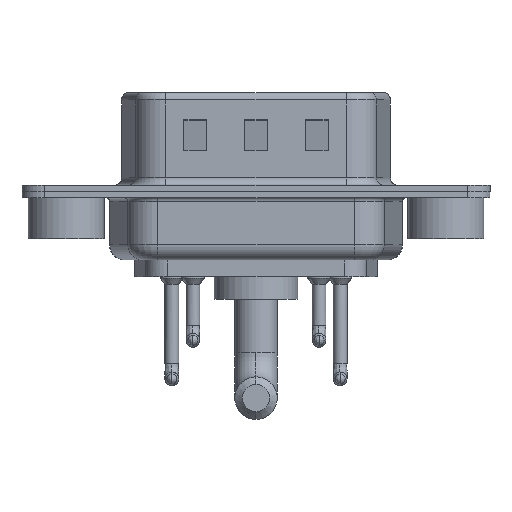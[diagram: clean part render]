
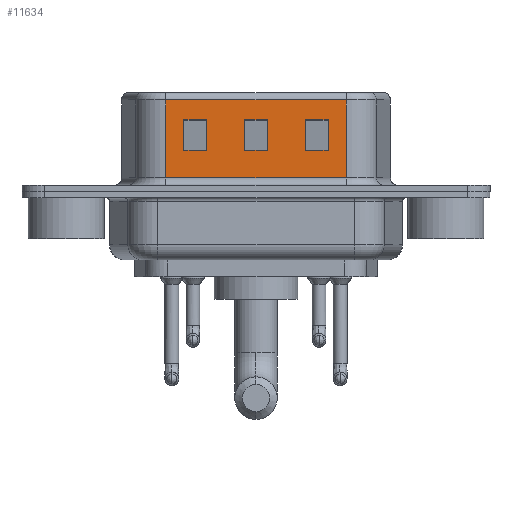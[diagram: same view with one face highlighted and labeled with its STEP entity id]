
A CAD part, front view. The second image highlights one B-rep face of the part: STEP entity #11634.
In plain terms, the highlighted planar face has unit normal (0, -1, 0).
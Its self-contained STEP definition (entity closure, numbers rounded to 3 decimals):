
#128 = EDGE_CURVE ( 'NONE', #5063, #8167, #14056, .T. ) ;
#356 = LINE ( 'NONE', #6371, #14150 ) ;
#477 = EDGE_CURVE ( 'NONE', #14121, #3612, #18324, .T. ) ;
#499 = EDGE_CURVE ( 'NONE', #4351, #4572, #15110, .T. ) ;
#601 = CARTESIAN_POINT ( 'NONE',  ( 14.451, -4.55, 2.705 ) ) ;
#802 = VERTEX_POINT ( 'NONE', #18299 ) ;
#902 = ORIENTED_EDGE ( 'NONE', *, *, #18445, .T. ) ;
#1031 = VERTEX_POINT ( 'NONE', #9601 ) ;
#1108 = CARTESIAN_POINT ( 'NONE',  ( 6.549, -4.55, 6.52 ) ) ;
#1173 = LINE ( 'NONE', #16094, #11653 ) ;
#1307 = VECTOR ( 'NONE', #13290, 1000. ) ;
#1339 = CARTESIAN_POINT ( 'NONE',  ( 9.25, -4.55, 2.705 ) ) ;
#1343 = ORIENTED_EDGE ( 'NONE', *, *, #5036, .T. ) ;
#1768 = ORIENTED_EDGE ( 'NONE', *, *, #6994, .T. ) ;
#1945 = VECTOR ( 'NONE', #11709, 1000. ) ;
#1950 = ORIENTED_EDGE ( 'NONE', *, *, #3753, .T. ) ;
#1970 = CARTESIAN_POINT ( 'NONE',  ( 17.25, -4.55, 2.705 ) ) ;
#2017 = CARTESIAN_POINT ( 'NONE',  ( 18.451, -4.55, 4.705 ) ) ;
#2020 = EDGE_LOOP ( 'NONE', ( #1343, #16700, #18065, #10295 ) ) ;
#2529 = CARTESIAN_POINT ( 'NONE',  ( 17.25, -4.55, 6.52 ) ) ;
#2638 = EDGE_CURVE ( 'NONE', #14281, #4351, #15765, .T. ) ;
#2662 = DIRECTION ( 'NONE',  ( -1., 0., 0. ) ) ;
#2970 = CARTESIAN_POINT ( 'NONE',  ( 6.549, -4.55, 6.02 ) ) ;
#3212 = DIRECTION ( 'NONE',  ( 1., 0., 0. ) ) ;
#3612 = VERTEX_POINT ( 'NONE', #17578 ) ;
#3753 = EDGE_CURVE ( 'NONE', #1031, #14281, #15665, .T. ) ;
#4274 = VECTOR ( 'NONE', #14164, 1000. ) ;
#4351 = VERTEX_POINT ( 'NONE', #9776 ) ;
#4566 = CARTESIAN_POINT ( 'NONE',  ( 13.25, -4.55, 4.705 ) ) ;
#4572 = VERTEX_POINT ( 'NONE', #4642 ) ;
#4622 = FACE_BOUND ( 'NONE', #5093, .T. ) ;
#4642 = CARTESIAN_POINT ( 'NONE',  ( 11.75, -4.55, 2.705 ) ) ;
#4907 = DIRECTION ( 'NONE',  ( 1., 0., 0. ) ) ;
#5036 = EDGE_CURVE ( 'NONE', #5867, #17017, #17137, .T. ) ;
#5063 = VERTEX_POINT ( 'NONE', #8634 ) ;
#5092 = DIRECTION ( 'NONE',  ( 0., 0., -1. ) ) ;
#5093 = EDGE_LOOP ( 'NONE', ( #1768, #17244, #14365, #19279 ) ) ;
#5263 = CARTESIAN_POINT ( 'NONE',  ( 22.451, -4.55, 4.705 ) ) ;
#5431 = CARTESIAN_POINT ( 'NONE',  ( 11.75, -4.55, 6.52 ) ) ;
#5535 = CARTESIAN_POINT ( 'NONE',  ( 18.451, -4.55, 6.02 ) ) ;
#5743 = ORIENTED_EDGE ( 'NONE', *, *, #2638, .T. ) ;
#5830 = FACE_OUTER_BOUND ( 'NONE', #16742, .T. ) ;
#5857 = AXIS2_PLACEMENT_3D ( 'NONE', #16572, #8868, #17960 ) ;
#5867 = VERTEX_POINT ( 'NONE', #17376 ) ;
#6016 = PLANE ( 'NONE',  #5857 ) ;
#6200 = DIRECTION ( 'NONE',  ( -1., 0., 0. ) ) ;
#6339 = VECTOR ( 'NONE', #15327, 1000. ) ;
#6349 = VERTEX_POINT ( 'NONE', #17640 ) ;
#6371 = CARTESIAN_POINT ( 'NONE',  ( 9.25, -4.55, 6.52 ) ) ;
#6527 = ORIENTED_EDGE ( 'NONE', *, *, #128, .T. ) ;
#6593 = ORIENTED_EDGE ( 'NONE', *, *, #10808, .F. ) ;
#6619 = DIRECTION ( 'NONE',  ( -1., 0., 0. ) ) ;
#6920 = VECTOR ( 'NONE', #13998, 1000. ) ;
#6994 = EDGE_CURVE ( 'NONE', #802, #10738, #356, .T. ) ;
#7208 = EDGE_CURVE ( 'NONE', #17017, #16033, #1173, .T. ) ;
#7352 = VECTOR ( 'NONE', #15344, 1000. ) ;
#7589 = FACE_BOUND ( 'NONE', #2020, .T. ) ;
#7590 = CARTESIAN_POINT ( 'NONE',  ( 18.451, -4.55, 0.9 ) ) ;
#7920 = EDGE_CURVE ( 'NONE', #10738, #10003, #12781, .T. ) ;
#8167 = VERTEX_POINT ( 'NONE', #2970 ) ;
#8634 = CARTESIAN_POINT ( 'NONE',  ( 18.451, -4.55, 6.02 ) ) ;
#8868 = DIRECTION ( 'NONE',  ( 0., 1., 0. ) ) ;
#9039 = VECTOR ( 'NONE', #9689, 1000. ) ;
#9170 = CARTESIAN_POINT ( 'NONE',  ( 15.75, -4.55, 6.52 ) ) ;
#9186 = CARTESIAN_POINT ( 'NONE',  ( 18.451, -4.55, 6.52 ) ) ;
#9601 = CARTESIAN_POINT ( 'NONE',  ( 11.75, -4.55, 4.705 ) ) ;
#9689 = DIRECTION ( 'NONE',  ( 0., 0., -1. ) ) ;
#9776 = CARTESIAN_POINT ( 'NONE',  ( 13.25, -4.55, 2.705 ) ) ;
#9869 = CARTESIAN_POINT ( 'NONE',  ( 15.75, -4.55, 4.705 ) ) ;
#10003 = VERTEX_POINT ( 'NONE', #17163 ) ;
#10171 = LINE ( 'NONE', #1108, #1307 ) ;
#10219 = ORIENTED_EDGE ( 'NONE', *, *, #477, .T. ) ;
#10240 = VECTOR ( 'NONE', #4907, 1000. ) ;
#10295 = ORIENTED_EDGE ( 'NONE', *, *, #10920, .T. ) ;
#10327 = LINE ( 'NONE', #5431, #1945 ) ;
#10393 = EDGE_CURVE ( 'NONE', #6349, #802, #15086, .T. ) ;
#10465 = CARTESIAN_POINT ( 'NONE',  ( 6.549, -4.55, 0.9 ) ) ;
#10635 = DIRECTION ( 'NONE',  ( 0., 0., 1. ) ) ;
#10738 = VERTEX_POINT ( 'NONE', #1339 ) ;
#10808 = EDGE_CURVE ( 'NONE', #5063, #3612, #12123, .T. ) ;
#10831 = LINE ( 'NONE', #16790, #6339 ) ;
#10920 = EDGE_CURVE ( 'NONE', #16696, #5867, #18279, .T. ) ;
#11634 = ADVANCED_FACE ( 'NONE', ( #4622, #7589, #13559, #5830 ), #6016, .F. ) ;
#11653 = VECTOR ( 'NONE', #2662, 1000. ) ;
#11709 = DIRECTION ( 'NONE',  ( 0., 0., 1. ) ) ;
#12123 = LINE ( 'NONE', #9186, #17005 ) ;
#12298 = LINE ( 'NONE', #9170, #15770 ) ;
#12690 = EDGE_CURVE ( 'NONE', #16033, #16696, #12298, .T. ) ;
#12781 = LINE ( 'NONE', #601, #14178 ) ;
#12993 = ORIENTED_EDGE ( 'NONE', *, *, #499, .T. ) ;
#13290 = DIRECTION ( 'NONE',  ( 0., 0., -1. ) ) ;
#13559 = FACE_BOUND ( 'NONE', #17424, .T. ) ;
#13574 = VECTOR ( 'NONE', #3212, 1000. ) ;
#13998 = DIRECTION ( 'NONE',  ( 1., 0., 0. ) ) ;
#14056 = LINE ( 'NONE', #5535, #4274 ) ;
#14121 = VERTEX_POINT ( 'NONE', #10465 ) ;
#14150 = VECTOR ( 'NONE', #5092, 1000. ) ;
#14164 = DIRECTION ( 'NONE',  ( -1., 0., 0. ) ) ;
#14178 = VECTOR ( 'NONE', #6619, 1000. ) ;
#14265 = EDGE_CURVE ( 'NONE', #10003, #6349, #10831, .T. ) ;
#14281 = VERTEX_POINT ( 'NONE', #4566 ) ;
#14365 = ORIENTED_EDGE ( 'NONE', *, *, #14265, .T. ) ;
#15002 = VECTOR ( 'NONE', #15676, 1000. ) ;
#15086 = LINE ( 'NONE', #16644, #13574 ) ;
#15110 = LINE ( 'NONE', #15201, #16157 ) ;
#15201 = CARTESIAN_POINT ( 'NONE',  ( 18.451, -4.55, 2.705 ) ) ;
#15327 = DIRECTION ( 'NONE',  ( 0., 0., 1. ) ) ;
#15344 = DIRECTION ( 'NONE',  ( 1., 0., 0. ) ) ;
#15665 = LINE ( 'NONE', #2017, #6920 ) ;
#15676 = DIRECTION ( 'NONE',  ( 0., 0., -1. ) ) ;
#15765 = LINE ( 'NONE', #18591, #9039 ) ;
#15770 = VECTOR ( 'NONE', #10635, 1000. ) ;
#16033 = VERTEX_POINT ( 'NONE', #17765 ) ;
#16094 = CARTESIAN_POINT ( 'NONE',  ( 22.451, -4.55, 2.705 ) ) ;
#16157 = VECTOR ( 'NONE', #6200, 1000. ) ;
#16572 = CARTESIAN_POINT ( 'NONE',  ( 18.451, -4.55, 6.52 ) ) ;
#16644 = CARTESIAN_POINT ( 'NONE',  ( 14.451, -4.55, 4.705 ) ) ;
#16696 = VERTEX_POINT ( 'NONE', #9869 ) ;
#16700 = ORIENTED_EDGE ( 'NONE', *, *, #7208, .T. ) ;
#16742 = EDGE_LOOP ( 'NONE', ( #6593, #6527, #902, #10219 ) ) ;
#16790 = CARTESIAN_POINT ( 'NONE',  ( 7.75, -4.55, 6.52 ) ) ;
#17005 = VECTOR ( 'NONE', #19273, 1000. ) ;
#17017 = VERTEX_POINT ( 'NONE', #1970 ) ;
#17137 = LINE ( 'NONE', #2529, #15002 ) ;
#17163 = CARTESIAN_POINT ( 'NONE',  ( 7.75, -4.55, 2.705 ) ) ;
#17244 = ORIENTED_EDGE ( 'NONE', *, *, #7920, .T. ) ;
#17376 = CARTESIAN_POINT ( 'NONE',  ( 17.25, -4.55, 4.705 ) ) ;
#17424 = EDGE_LOOP ( 'NONE', ( #1950, #5743, #12993, #19149 ) ) ;
#17578 = CARTESIAN_POINT ( 'NONE',  ( 18.451, -4.55, 0.9 ) ) ;
#17640 = CARTESIAN_POINT ( 'NONE',  ( 7.75, -4.55, 4.705 ) ) ;
#17765 = CARTESIAN_POINT ( 'NONE',  ( 15.75, -4.55, 2.705 ) ) ;
#17960 = DIRECTION ( 'NONE',  ( -1., 0., 0. ) ) ;
#18065 = ORIENTED_EDGE ( 'NONE', *, *, #12690, .T. ) ;
#18279 = LINE ( 'NONE', #5263, #7352 ) ;
#18299 = CARTESIAN_POINT ( 'NONE',  ( 9.25, -4.55, 4.705 ) ) ;
#18324 = LINE ( 'NONE', #7590, #10240 ) ;
#18445 = EDGE_CURVE ( 'NONE', #8167, #14121, #10171, .T. ) ;
#18591 = CARTESIAN_POINT ( 'NONE',  ( 13.25, -4.55, 6.52 ) ) ;
#18847 = EDGE_CURVE ( 'NONE', #4572, #1031, #10327, .T. ) ;
#19149 = ORIENTED_EDGE ( 'NONE', *, *, #18847, .T. ) ;
#19273 = DIRECTION ( 'NONE',  ( 0., 0., -1. ) ) ;
#19279 = ORIENTED_EDGE ( 'NONE', *, *, #10393, .T. ) ;
